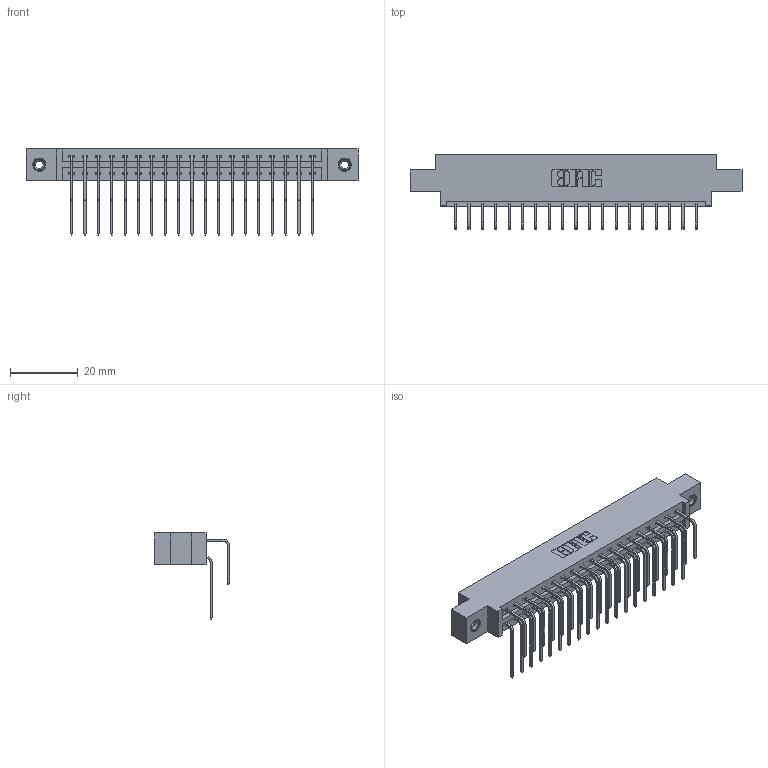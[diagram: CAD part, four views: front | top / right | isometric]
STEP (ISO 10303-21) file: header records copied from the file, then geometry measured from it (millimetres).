
FILE_DESCRIPTION (( 'STEP AP203' ), '1' );
FILE_NAME ('387-038-558-808.STEP', '2018-09-19T06:46:46', ( '' ), ( '' ), 'SwSTEP 2.0', 'SolidWorks 2016', '' );
FILE_SCHEMA (( 'CONFIG_CONTROL_DESIGN' ));
Length unit declared in the file: inch
Products named in the file (5): 345-292-001_558 559 Tail - 1; 345-292-001_558 Tail - 2; 345-250-001_345-250-003-102; 387-038-558-808; 337 Part_0.170 Offset - 0.156 Dia-TI
Assembly tree (41 placements, depth 2):
  387-038-558-808
    337 Part_0.170 Offset - 0.156 Dia-TI
    345-292-001_558 559 Tail - 1  x19
    345-292-001_558 Tail - 2  x19
    345-250-001_345-250-003-102  x2
Bounding box: 98.3 x 22.17 x 25.53 mm (x, y, z)
Volume: 10148.5 mm3; surface area: 12481.9 mm2
Topology: 41 solids, 41 shells, 2306 faces, 6805 edges, 4478 vertices
Faces by surface type: plane 1626, cylinder 664, cone 12, torus 4
Entity records: 20808 total; most frequent: CARTESIAN_POINT 3552, ORIENTED_EDGE 3430, DIRECTION 3077, EDGE_CURVE 1715, VECTOR 1527, LINE 1527, VERTEX_POINT 1136, AXIS2_PLACEMENT_3D 775
